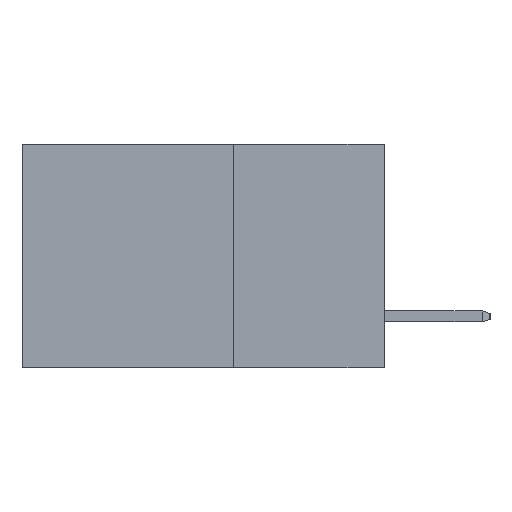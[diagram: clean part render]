
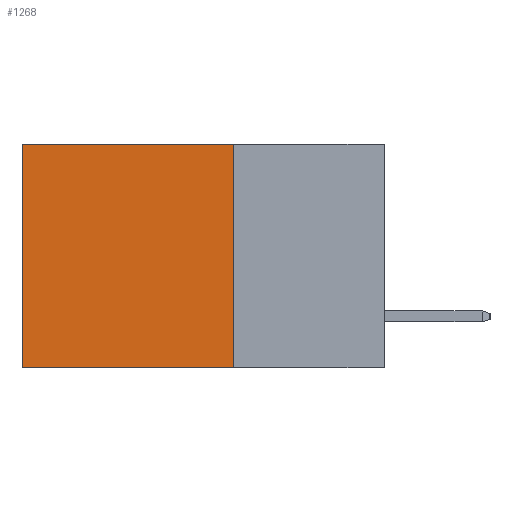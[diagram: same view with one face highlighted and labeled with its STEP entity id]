
A CAD part, left-side view. The second image highlights one B-rep face of the part: STEP entity #1268.
In plain terms, the highlighted planar face has unit normal (-1, 0, 0).
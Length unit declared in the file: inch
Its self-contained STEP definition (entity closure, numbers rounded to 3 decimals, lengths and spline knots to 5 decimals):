
#1268 = ADVANCED_FACE ( 'NONE', ( #20776 ), #18127, .F. ) ;
#2438 = EDGE_CURVE ( 'NONE', #19094, #11778, #7316, .T. ) ;
#2553 = LINE ( 'NONE', #6698, #10953 ) ;
#2855 = ORIENTED_EDGE ( 'NONE', *, *, #11989, .T. ) ;
#4649 = VECTOR ( 'NONE', #7605, 39.37008 ) ;
#5036 = CARTESIAN_POINT ( 'NONE',  ( 0.2615, 0.25, -0.37 ) ) ;
#5591 = DIRECTION ( 'NONE',  ( 0., 1., 0. ) ) ;
#5787 = CARTESIAN_POINT ( 'NONE',  ( 0.2615, 0.25, -0.37 ) ) ;
#6698 = CARTESIAN_POINT ( 'NONE',  ( 0.2615, 0.6, -0.37 ) ) ;
#6776 = AXIS2_PLACEMENT_3D ( 'NONE', #15463, #17061, #17039 ) ;
#6960 = DIRECTION ( 'NONE',  ( 0., 0., -1. ) ) ;
#7316 = LINE ( 'NONE', #5036, #19549 ) ;
#7605 = DIRECTION ( 'NONE',  ( 0., 1., 0. ) ) ;
#7717 = EDGE_CURVE ( 'NONE', #12699, #19677, #13932, .T. ) ;
#7831 = CARTESIAN_POINT ( 'NONE',  ( 0.2615, 0.25, 0. ) ) ;
#10194 = LINE ( 'NONE', #5787, #14418 ) ;
#10953 = VECTOR ( 'NONE', #6960, 39.37008 ) ;
#11778 = VERTEX_POINT ( 'NONE', #17154 ) ;
#11989 = EDGE_CURVE ( 'NONE', #19677, #11778, #2553, .T. ) ;
#12699 = VERTEX_POINT ( 'NONE', #13064 ) ;
#13064 = CARTESIAN_POINT ( 'NONE',  ( 0.2615, 0.25, 0. ) ) ;
#13327 = EDGE_LOOP ( 'NONE', ( #2855, #19173, #17695, #13781 ) ) ;
#13781 = ORIENTED_EDGE ( 'NONE', *, *, #7717, .T. ) ;
#13932 = LINE ( 'NONE', #7831, #4649 ) ;
#13965 = DIRECTION ( 'NONE',  ( 0., 0., -1. ) ) ;
#14418 = VECTOR ( 'NONE', #13965, 39.37008 ) ;
#15463 = CARTESIAN_POINT ( 'NONE',  ( 0.2615, 0.25, -0.37 ) ) ;
#16078 = CARTESIAN_POINT ( 'NONE',  ( 0.2615, 0.25, -0.37 ) ) ;
#17039 = DIRECTION ( 'NONE',  ( 0., 0., -1. ) ) ;
#17061 = DIRECTION ( 'NONE',  ( 1., 0., 0. ) ) ;
#17154 = CARTESIAN_POINT ( 'NONE',  ( 0.2615, 0.6, -0.37 ) ) ;
#17359 = CARTESIAN_POINT ( 'NONE',  ( 0.2615, 0.6, 0. ) ) ;
#17695 = ORIENTED_EDGE ( 'NONE', *, *, #19576, .F. ) ;
#18127 = PLANE ( 'NONE',  #6776 ) ;
#19094 = VERTEX_POINT ( 'NONE', #16078 ) ;
#19173 = ORIENTED_EDGE ( 'NONE', *, *, #2438, .F. ) ;
#19549 = VECTOR ( 'NONE', #5591, 39.37008 ) ;
#19576 = EDGE_CURVE ( 'NONE', #12699, #19094, #10194, .T. ) ;
#19677 = VERTEX_POINT ( 'NONE', #17359 ) ;
#20776 = FACE_OUTER_BOUND ( 'NONE', #13327, .T. ) ;
